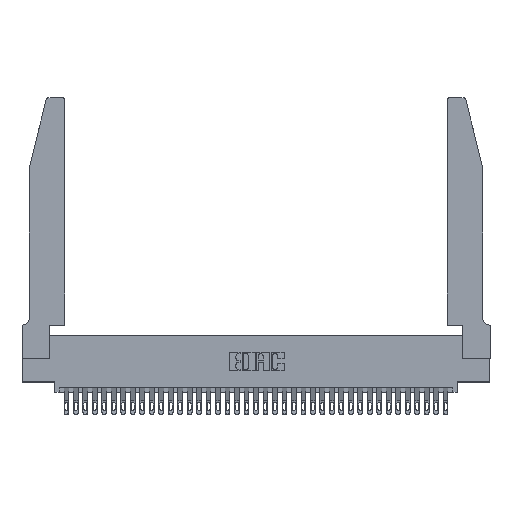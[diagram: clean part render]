
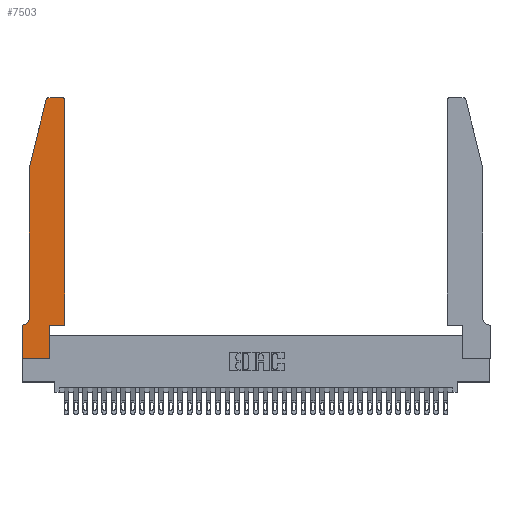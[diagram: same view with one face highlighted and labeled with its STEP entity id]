
A CAD part, top view. The second image highlights one B-rep face of the part: STEP entity #7503.
In plain terms, the highlighted planar face has unit normal (0, 0, 1).
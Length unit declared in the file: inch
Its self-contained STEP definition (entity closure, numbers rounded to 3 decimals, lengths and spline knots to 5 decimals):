
#204 = EDGE_CURVE ( 'NONE', #1670, #20804, #13305, .T. ) ;
#211 = CIRCLE ( 'NONE', #24058, 0.03 ) ;
#233 = ORIENTED_EDGE ( 'NONE', *, *, #204, .T. ) ;
#344 = CARTESIAN_POINT ( 'NONE',  ( 0.4505, 0.35, 0.37 ) ) ;
#808 = CARTESIAN_POINT ( 'NONE',  ( 0.0755, 2., 0.37 ) ) ;
#935 = DIRECTION ( 'NONE',  ( -1., 0., 0. ) ) ;
#1175 = ORIENTED_EDGE ( 'NONE', *, *, #18382, .T. ) ;
#1185 = VECTOR ( 'NONE', #13334, 39.37008 ) ;
#1612 = CARTESIAN_POINT ( 'NONE',  ( 0., 0.35, 0.37 ) ) ;
#1670 = VERTEX_POINT ( 'NONE', #36286 ) ;
#2176 = EDGE_LOOP ( 'NONE', ( #15963, #233, #1175, #2935, #3049, #8214, #7524, #8352, #18878, #28805, #20344, #10845 ) ) ;
#2282 = VERTEX_POINT ( 'NONE', #24699 ) ;
#2700 = DIRECTION ( 'NONE',  ( 0., 0., -1. ) ) ;
#2918 = DIRECTION ( 'NONE',  ( 0., 1., 0. ) ) ;
#2935 = ORIENTED_EDGE ( 'NONE', *, *, #34880, .T. ) ;
#3049 = ORIENTED_EDGE ( 'NONE', *, *, #7024, .T. ) ;
#3309 = CARTESIAN_POINT ( 'NONE',  ( 0.284, 2.72, 0.37 ) ) ;
#3845 = DIRECTION ( 'NONE',  ( 0., -1., 0. ) ) ;
#3988 = VERTEX_POINT ( 'NONE', #4405 ) ;
#4302 = CARTESIAN_POINT ( 'NONE',  ( 0.4505, 2.72, 0.37 ) ) ;
#4405 = CARTESIAN_POINT ( 'NONE',  ( 0.0755, 2., 0.37 ) ) ;
#4833 = CIRCLE ( 'NONE', #15449, 0.07 ) ;
#5263 = LINE ( 'NONE', #35943, #19003 ) ;
#5408 = CARTESIAN_POINT ( 'NONE',  ( 0.4505, 0.35, 0.37 ) ) ;
#5754 = VECTOR ( 'NONE', #20953, 39.37008 ) ;
#5755 = EDGE_CURVE ( 'NONE', #33740, #7518, #211, .T. ) ;
#6346 = DIRECTION ( 'NONE',  ( 1., 0., 0. ) ) ;
#7024 = EDGE_CURVE ( 'NONE', #11815, #21357, #4833, .T. ) ;
#7349 = CARTESIAN_POINT ( 'NONE',  ( 0., 0., 0.37 ) ) ;
#7503 = ADVANCED_FACE ( 'NONE', ( #27918 ), #25108, .T. ) ;
#7518 = VERTEX_POINT ( 'NONE', #16617 ) ;
#7524 = ORIENTED_EDGE ( 'NONE', *, *, #37276, .T. ) ;
#7973 = CARTESIAN_POINT ( 'NONE',  ( 0.0055, 0.35, 0.37 ) ) ;
#8133 = CARTESIAN_POINT ( 'NONE',  ( 0.0755, 0.35, 0.37 ) ) ;
#8214 = ORIENTED_EDGE ( 'NONE', *, *, #24756, .T. ) ;
#8352 = ORIENTED_EDGE ( 'NONE', *, *, #33747, .T. ) ;
#9806 = CARTESIAN_POINT ( 'NONE',  ( 0.4205, 2.72, 0.37 ) ) ;
#10704 = VECTOR ( 'NONE', #2918, 39.37008 ) ;
#10785 = DIRECTION ( 'NONE',  ( 1., 0., 0. ) ) ;
#10845 = ORIENTED_EDGE ( 'NONE', *, *, #5755, .T. ) ;
#11815 = VERTEX_POINT ( 'NONE', #28229 ) ;
#12757 = DIRECTION ( 'NONE',  ( 1., 0., 0. ) ) ;
#12967 = VERTEX_POINT ( 'NONE', #25657 ) ;
#13305 = CIRCLE ( 'NONE', #34857, 0.03 ) ;
#13334 = DIRECTION ( 'NONE',  ( -0.239, -0.971, 0. ) ) ;
#14732 = DIRECTION ( 'NONE',  ( 0., -1., 0. ) ) ;
#15449 = AXIS2_PLACEMENT_3D ( 'NONE', #20301, #2700, #23155 ) ;
#15725 = CARTESIAN_POINT ( 'NONE',  ( 0.2605, 2.75, 0.37 ) ) ;
#15771 = CARTESIAN_POINT ( 'NONE',  ( 0.2865, 0., 0.37 ) ) ;
#15963 = ORIENTED_EDGE ( 'NONE', *, *, #29076, .T. ) ;
#16292 = LINE ( 'NONE', #7349, #23022 ) ;
#16617 = CARTESIAN_POINT ( 'NONE',  ( 0.4205, 2.75, 0.37 ) ) ;
#16715 = EDGE_CURVE ( 'NONE', #31326, #31974, #17504, .T. ) ;
#17504 = LINE ( 'NONE', #17616, #10704 ) ;
#17616 = CARTESIAN_POINT ( 'NONE',  ( 0.2865, 0.35, 0.37 ) ) ;
#18382 = EDGE_CURVE ( 'NONE', #20804, #3988, #32094, .T. ) ;
#18878 = ORIENTED_EDGE ( 'NONE', *, *, #16715, .T. ) ;
#19003 = VECTOR ( 'NONE', #21811, 39.37008 ) ;
#20301 = CARTESIAN_POINT ( 'NONE',  ( 0.0055, 0.42, 0.37 ) ) ;
#20344 = ORIENTED_EDGE ( 'NONE', *, *, #25246, .T. ) ;
#20787 = LINE ( 'NONE', #31819, #36777 ) ;
#20804 = VERTEX_POINT ( 'NONE', #32882 ) ;
#20953 = DIRECTION ( 'NONE',  ( 1., 0., 0. ) ) ;
#21357 = VERTEX_POINT ( 'NONE', #7973 ) ;
#21811 = DIRECTION ( 'NONE',  ( 0., 1., 0. ) ) ;
#23022 = VECTOR ( 'NONE', #33248, 39.37008 ) ;
#23155 = DIRECTION ( 'NONE',  ( -1., 0., 0. ) ) ;
#23728 = DIRECTION ( 'NONE',  ( 0., 0., 1. ) ) ;
#24058 = AXIS2_PLACEMENT_3D ( 'NONE', #9806, #29867, #12757 ) ;
#24251 = CARTESIAN_POINT ( 'NONE',  ( 0.2865, 0.35, 0.37 ) ) ;
#24699 = CARTESIAN_POINT ( 'NONE',  ( 0., 0.35, 0.37 ) ) ;
#24756 = EDGE_CURVE ( 'NONE', #21357, #2282, #36330, .T. ) ;
#25036 = EDGE_CURVE ( 'NONE', #31974, #27412, #34600, .T. ) ;
#25108 = PLANE ( 'NONE',  #35735 ) ;
#25246 = EDGE_CURVE ( 'NONE', #27412, #33740, #5263, .T. ) ;
#25657 = CARTESIAN_POINT ( 'NONE',  ( 0., 0., 0.37 ) ) ;
#25791 = LINE ( 'NONE', #808, #32964 ) ;
#27412 = VERTEX_POINT ( 'NONE', #5408 ) ;
#27559 = CARTESIAN_POINT ( 'NONE',  ( 0.0755, 2., 0.37 ) ) ;
#27918 = FACE_OUTER_BOUND ( 'NONE', #2176, .T. ) ;
#27950 = DIRECTION ( 'NONE',  ( 0., 0., 1. ) ) ;
#28229 = CARTESIAN_POINT ( 'NONE',  ( 0.0755, 0.42, 0.37 ) ) ;
#28805 = ORIENTED_EDGE ( 'NONE', *, *, #25036, .T. ) ;
#29076 = EDGE_CURVE ( 'NONE', #7518, #1670, #29082, .T. ) ;
#29082 = LINE ( 'NONE', #15725, #35767 ) ;
#29867 = DIRECTION ( 'NONE',  ( 0., 0., 1. ) ) ;
#31326 = VERTEX_POINT ( 'NONE', #15771 ) ;
#31819 = CARTESIAN_POINT ( 'NONE',  ( 0., 0., 0.37 ) ) ;
#31974 = VERTEX_POINT ( 'NONE', #24251 ) ;
#32094 = LINE ( 'NONE', #27559, #1185 ) ;
#32882 = CARTESIAN_POINT ( 'NONE',  ( 0.25487, 2.72718, 0.37 ) ) ;
#32964 = VECTOR ( 'NONE', #3845, 39.37008 ) ;
#33248 = DIRECTION ( 'NONE',  ( 1., 0., 0. ) ) ;
#33740 = VERTEX_POINT ( 'NONE', #4302 ) ;
#33747 = EDGE_CURVE ( 'NONE', #12967, #31326, #16292, .T. ) ;
#34600 = LINE ( 'NONE', #344, #5754 ) ;
#34857 = AXIS2_PLACEMENT_3D ( 'NONE', #3309, #23728, #6346 ) ;
#34880 = EDGE_CURVE ( 'NONE', #3988, #11815, #25791, .T. ) ;
#35735 = AXIS2_PLACEMENT_3D ( 'NONE', #1612, #27950, #10785 ) ;
#35767 = VECTOR ( 'NONE', #935, 39.37008 ) ;
#35943 = CARTESIAN_POINT ( 'NONE',  ( 0.4505, 0.35, 0.37 ) ) ;
#36286 = CARTESIAN_POINT ( 'NONE',  ( 0.284, 2.75, 0.37 ) ) ;
#36330 = LINE ( 'NONE', #8133, #37234 ) ;
#36727 = DIRECTION ( 'NONE',  ( -1., 0., 0. ) ) ;
#36777 = VECTOR ( 'NONE', #14732, 39.37008 ) ;
#37234 = VECTOR ( 'NONE', #36727, 39.37008 ) ;
#37276 = EDGE_CURVE ( 'NONE', #2282, #12967, #20787, .T. ) ;
